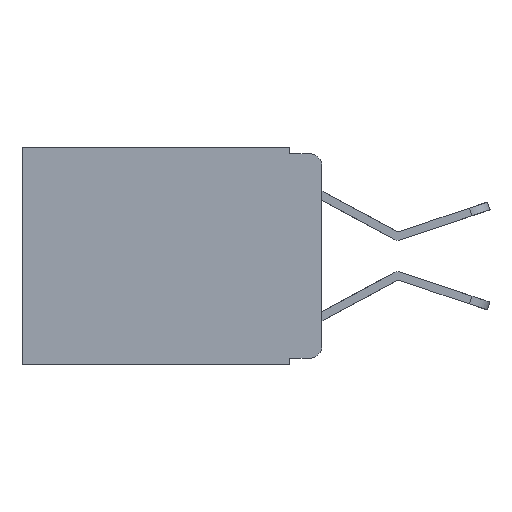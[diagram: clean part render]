
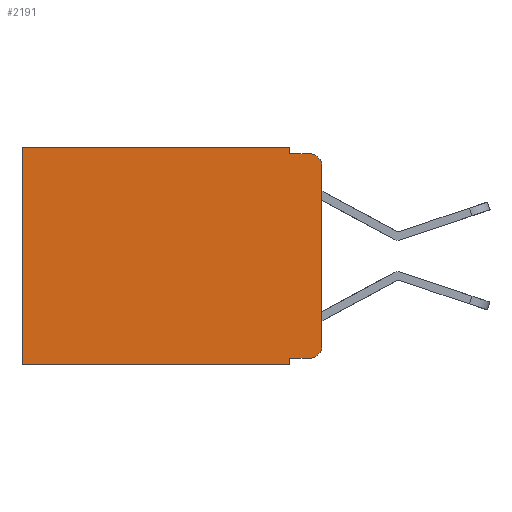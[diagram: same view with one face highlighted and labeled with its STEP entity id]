
A CAD part, left-side view. The second image highlights one B-rep face of the part: STEP entity #2191.
In plain terms, the highlighted planar face has unit normal (-1, 0, 0).
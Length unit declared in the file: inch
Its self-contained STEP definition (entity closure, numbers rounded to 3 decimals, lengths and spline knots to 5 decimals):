
#47 = ORIENTED_EDGE ( 'NONE', *, *, #15987, .T. ) ;
#633 = VERTEX_POINT ( 'NONE', #12923 ) ;
#688 = LINE ( 'NONE', #6027, #3922 ) ;
#1086 = EDGE_CURVE ( 'NONE', #12166, #2786, #18721, .T. ) ;
#1344 = VERTEX_POINT ( 'NONE', #13216 ) ;
#1747 = DIRECTION ( 'NONE',  ( 0., 0., -1. ) ) ;
#1806 = VECTOR ( 'NONE', #13198, 39.37008 ) ;
#1914 = VECTOR ( 'NONE', #19055, 39.37008 ) ;
#2009 = VERTEX_POINT ( 'NONE', #4046 ) ;
#2191 = ADVANCED_FACE ( 'NONE', ( #16589 ), #2802, .F. ) ;
#2245 = VECTOR ( 'NONE', #4930, 39.37008 ) ;
#2332 = CARTESIAN_POINT ( 'NONE',  ( 0.298, 0.473, -0.343 ) ) ;
#2786 = VERTEX_POINT ( 'NONE', #5848 ) ;
#2802 = PLANE ( 'NONE',  #17549 ) ;
#3007 = ORIENTED_EDGE ( 'NONE', *, *, #18450, .F. ) ;
#3343 = CARTESIAN_POINT ( 'NONE',  ( 0.298, 0.473, 0. ) ) ;
#3553 = CARTESIAN_POINT ( 'NONE',  ( 0.298, 0., -0.343 ) ) ;
#3922 = VECTOR ( 'NONE', #15207, 39.37008 ) ;
#4046 = CARTESIAN_POINT ( 'NONE',  ( 0.298, 0.02, -0.333 ) ) ;
#4068 = VECTOR ( 'NONE', #1747, 39.37008 ) ;
#4118 = DIRECTION ( 'NONE',  ( 0., 0., -1. ) ) ;
#4315 = DIRECTION ( 'NONE',  ( 0., 0., -1. ) ) ;
#4365 = EDGE_CURVE ( 'NONE', #633, #13588, #12342, .T. ) ;
#4728 = DIRECTION ( 'NONE',  ( -1., 0., 0. ) ) ;
#4772 = LINE ( 'NONE', #11882, #12529 ) ;
#4874 = CARTESIAN_POINT ( 'NONE',  ( 0.298, 0., 0. ) ) ;
#4912 = CARTESIAN_POINT ( 'NONE',  ( 0.298, 0.051, -0.343 ) ) ;
#4930 = DIRECTION ( 'NONE',  ( 0., 0., -1. ) ) ;
#4959 = ORIENTED_EDGE ( 'NONE', *, *, #18022, .F. ) ;
#5088 = ORIENTED_EDGE ( 'NONE', *, *, #17026, .T. ) ;
#5248 = LINE ( 'NONE', #3553, #13453 ) ;
#5342 = EDGE_CURVE ( 'NONE', #633, #2786, #7750, .T. ) ;
#5543 = ORIENTED_EDGE ( 'NONE', *, *, #13362, .F. ) ;
#5613 = CARTESIAN_POINT ( 'NONE',  ( 0.298, 0.051, -0.01 ) ) ;
#5848 = CARTESIAN_POINT ( 'NONE',  ( 0.298, 0.02, -0.01 ) ) ;
#6027 = CARTESIAN_POINT ( 'NONE',  ( 0.298, 0.051, 0. ) ) ;
#6314 = ORIENTED_EDGE ( 'NONE', *, *, #16298, .T. ) ;
#6591 = VECTOR ( 'NONE', #16968, 39.37008 ) ;
#6915 = CARTESIAN_POINT ( 'NONE',  ( 0.298, 0., 0. ) ) ;
#7250 = AXIS2_PLACEMENT_3D ( 'NONE', #18011, #8939, #19480 ) ;
#7750 = CIRCLE ( 'NONE', #7250, 0.02 ) ;
#7870 = CIRCLE ( 'NONE', #14960, 0.02 ) ;
#8939 = DIRECTION ( 'NONE',  ( -1., 0., 0. ) ) ;
#10163 = VERTEX_POINT ( 'NONE', #4912 ) ;
#10263 = LINE ( 'NONE', #6915, #1914 ) ;
#10315 = ORIENTED_EDGE ( 'NONE', *, *, #4365, .F. ) ;
#10840 = CARTESIAN_POINT ( 'NONE',  ( 0.298, 0.051, -0.01 ) ) ;
#11433 = DIRECTION ( 'NONE',  ( 1., 0., 0. ) ) ;
#11698 = CARTESIAN_POINT ( 'NONE',  ( 0.298, 0.051, -0.333 ) ) ;
#11882 = CARTESIAN_POINT ( 'NONE',  ( 0.298, 0.051, 0. ) ) ;
#12051 = CARTESIAN_POINT ( 'NONE',  ( 0.298, 0., -0.313 ) ) ;
#12166 = VERTEX_POINT ( 'NONE', #5613 ) ;
#12342 = LINE ( 'NONE', #4874, #4068 ) ;
#12405 = CARTESIAN_POINT ( 'NONE',  ( 0.298, 0., 0. ) ) ;
#12529 = VECTOR ( 'NONE', #4118, 39.37008 ) ;
#12856 = DIRECTION ( 'NONE',  ( 0., 1., 0. ) ) ;
#12923 = CARTESIAN_POINT ( 'NONE',  ( 0.298, 0., -0.03 ) ) ;
#13198 = DIRECTION ( 'NONE',  ( 0., -1., 0. ) ) ;
#13216 = CARTESIAN_POINT ( 'NONE',  ( 0.298, 0.473, 0. ) ) ;
#13362 = EDGE_CURVE ( 'NONE', #19024, #12166, #688, .T. ) ;
#13453 = VECTOR ( 'NONE', #12856, 39.37008 ) ;
#13518 = CARTESIAN_POINT ( 'NONE',  ( 0.298, 0.051, -0.333 ) ) ;
#13588 = VERTEX_POINT ( 'NONE', #12051 ) ;
#13984 = CARTESIAN_POINT ( 'NONE',  ( 0.298, 0.02, -0.313 ) ) ;
#14126 = ORIENTED_EDGE ( 'NONE', *, *, #5342, .T. ) ;
#14206 = LINE ( 'NONE', #11698, #1806 ) ;
#14602 = ORIENTED_EDGE ( 'NONE', *, *, #1086, .F. ) ;
#14627 = LINE ( 'NONE', #3343, #2245 ) ;
#14960 = AXIS2_PLACEMENT_3D ( 'NONE', #13984, #4728, #15502 ) ;
#15207 = DIRECTION ( 'NONE',  ( 0., 0., -1. ) ) ;
#15326 = ORIENTED_EDGE ( 'NONE', *, *, #18996, .T. ) ;
#15502 = DIRECTION ( 'NONE',  ( 0., 0., -1. ) ) ;
#15731 = CARTESIAN_POINT ( 'NONE',  ( 0.298, 0.051, 0. ) ) ;
#15825 = VERTEX_POINT ( 'NONE', #13518 ) ;
#15875 = EDGE_LOOP ( 'NONE', ( #10315, #14126, #14602, #5543, #6314, #15326, #3007, #4959, #5088, #47 ) ) ;
#15987 = EDGE_CURVE ( 'NONE', #2009, #13588, #7870, .T. ) ;
#16298 = EDGE_CURVE ( 'NONE', #19024, #1344, #10263, .T. ) ;
#16589 = FACE_OUTER_BOUND ( 'NONE', #15875, .T. ) ;
#16968 = DIRECTION ( 'NONE',  ( 0., -1., 0. ) ) ;
#17026 = EDGE_CURVE ( 'NONE', #15825, #2009, #14206, .T. ) ;
#17037 = VERTEX_POINT ( 'NONE', #2332 ) ;
#17549 = AXIS2_PLACEMENT_3D ( 'NONE', #12405, #11433, #4315 ) ;
#18011 = CARTESIAN_POINT ( 'NONE',  ( 0.298, 0.02, -0.03 ) ) ;
#18022 = EDGE_CURVE ( 'NONE', #15825, #10163, #4772, .T. ) ;
#18450 = EDGE_CURVE ( 'NONE', #10163, #17037, #5248, .T. ) ;
#18721 = LINE ( 'NONE', #10840, #6591 ) ;
#18996 = EDGE_CURVE ( 'NONE', #1344, #17037, #14627, .T. ) ;
#19024 = VERTEX_POINT ( 'NONE', #15731 ) ;
#19055 = DIRECTION ( 'NONE',  ( 0., 1., 0. ) ) ;
#19480 = DIRECTION ( 'NONE',  ( 0., 0., -1. ) ) ;
